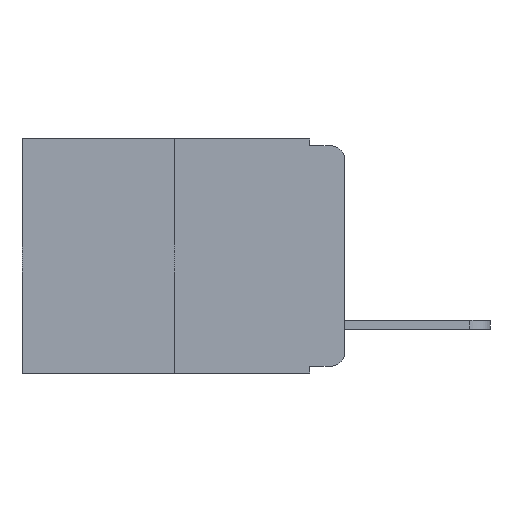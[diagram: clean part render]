
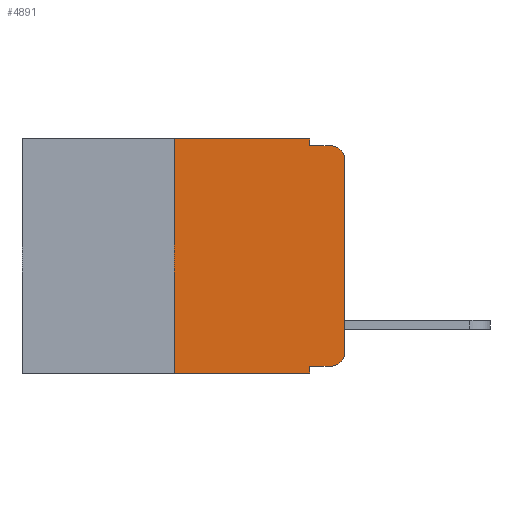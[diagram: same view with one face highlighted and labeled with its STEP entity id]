
A CAD part, left-side view. The second image highlights one B-rep face of the part: STEP entity #4891.
In plain terms, the highlighted planar face has unit normal (-1, 0, 0).
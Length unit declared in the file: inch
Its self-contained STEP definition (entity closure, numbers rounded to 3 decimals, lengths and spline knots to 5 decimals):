
#204 = LINE ( 'NONE', #1034, #8869 ) ;
#365 = EDGE_CURVE ( 'NONE', #8021, #4983, #11713, .T. ) ;
#414 = CARTESIAN_POINT ( 'NONE',  ( 0., 0., -0.313 ) ) ;
#567 = VECTOR ( 'NONE', #9850, 39.37008 ) ;
#837 = DIRECTION ( 'NONE',  ( -1., 0., 0. ) ) ;
#911 = VERTEX_POINT ( 'NONE', #12337 ) ;
#989 = VERTEX_POINT ( 'NONE', #10627 ) ;
#1034 = CARTESIAN_POINT ( 'NONE',  ( 0., 0.051, 0. ) ) ;
#1193 = ORIENTED_EDGE ( 'NONE', *, *, #3499, .T. ) ;
#1204 = EDGE_CURVE ( 'NONE', #8021, #5911, #12132, .T. ) ;
#1259 = PLANE ( 'NONE',  #11285 ) ;
#1434 = CARTESIAN_POINT ( 'NONE',  ( 0., 0.25, 0. ) ) ;
#1469 = ORIENTED_EDGE ( 'NONE', *, *, #8267, .T. ) ;
#1662 = DIRECTION ( 'NONE',  ( 0., -1., 0. ) ) ;
#1943 = CARTESIAN_POINT ( 'NONE',  ( 0., 0.473, 0. ) ) ;
#2091 = EDGE_CURVE ( 'NONE', #2557, #2866, #5139, .T. ) ;
#2169 = EDGE_CURVE ( 'NONE', #911, #7665, #3894, .T. ) ;
#2333 = DIRECTION ( 'NONE',  ( 1., 0., 0. ) ) ;
#2357 = EDGE_CURVE ( 'NONE', #7665, #2866, #12387, .T. ) ;
#2400 = DIRECTION ( 'NONE',  ( 0., 0., -1. ) ) ;
#2557 = VERTEX_POINT ( 'NONE', #4810 ) ;
#2712 = DIRECTION ( 'NONE',  ( 0., 0., -1. ) ) ;
#2798 = CARTESIAN_POINT ( 'NONE',  ( 0., 0., 0. ) ) ;
#2844 = VERTEX_POINT ( 'NONE', #4888 ) ;
#2866 = VERTEX_POINT ( 'NONE', #8182 ) ;
#3059 = CARTESIAN_POINT ( 'NONE',  ( 0., 0.25, 0. ) ) ;
#3358 = EDGE_CURVE ( 'NONE', #989, #2844, #4215, .T. ) ;
#3454 = EDGE_CURVE ( 'NONE', #989, #5911, #204, .T. ) ;
#3499 = EDGE_CURVE ( 'NONE', #2844, #7478, #7286, .T. ) ;
#3604 = CARTESIAN_POINT ( 'NONE',  ( 0., 0.051, -0.333 ) ) ;
#3894 = LINE ( 'NONE', #11073, #6180 ) ;
#4009 = CARTESIAN_POINT ( 'NONE',  ( 0., 0.473, -0.343 ) ) ;
#4024 = ORIENTED_EDGE ( 'NONE', *, *, #2357, .F. ) ;
#4215 = LINE ( 'NONE', #3604, #11380 ) ;
#4264 = VECTOR ( 'NONE', #5029, 39.37008 ) ;
#4461 = ORIENTED_EDGE ( 'NONE', *, *, #3358, .T. ) ;
#4555 = AXIS2_PLACEMENT_3D ( 'NONE', #12685, #11218, #11183 ) ;
#4810 = CARTESIAN_POINT ( 'NONE',  ( 0., 0., -0.03 ) ) ;
#4888 = CARTESIAN_POINT ( 'NONE',  ( 0., 0.02, -0.333 ) ) ;
#4891 = ADVANCED_FACE ( 'NONE', ( #7120 ), #1259, .F. ) ;
#4983 = VERTEX_POINT ( 'NONE', #1434 ) ;
#5029 = DIRECTION ( 'NONE',  ( 0., 0., 1. ) ) ;
#5051 = EDGE_LOOP ( 'NONE', ( #1469, #9804, #4024, #10085, #11496, #10766, #11885, #12178, #4461, #1193 ) ) ;
#5139 = CIRCLE ( 'NONE', #4555, 0.02 ) ;
#5370 = DIRECTION ( 'NONE',  ( 0., 0., -1. ) ) ;
#5911 = VERTEX_POINT ( 'NONE', #7107 ) ;
#5940 = LINE ( 'NONE', #2798, #567 ) ;
#6180 = VECTOR ( 'NONE', #5370, 39.37008 ) ;
#6460 = CARTESIAN_POINT ( 'NONE',  ( 0., 0.051, -0.01 ) ) ;
#6569 = AXIS2_PLACEMENT_3D ( 'NONE', #12702, #837, #2712 ) ;
#6968 = DIRECTION ( 'NONE',  ( 0., 0., -1. ) ) ;
#6973 = VECTOR ( 'NONE', #10863, 39.37008 ) ;
#6994 = VECTOR ( 'NONE', #10734, 39.37008 ) ;
#7107 = CARTESIAN_POINT ( 'NONE',  ( 0., 0.051, -0.343 ) ) ;
#7120 = FACE_OUTER_BOUND ( 'NONE', #5051, .T. ) ;
#7286 = CIRCLE ( 'NONE', #6569, 0.02 ) ;
#7478 = VERTEX_POINT ( 'NONE', #414 ) ;
#7665 = VERTEX_POINT ( 'NONE', #8048 ) ;
#8021 = VERTEX_POINT ( 'NONE', #10284 ) ;
#8048 = CARTESIAN_POINT ( 'NONE',  ( 0., 0.051, -0.01 ) ) ;
#8081 = DIRECTION ( 'NONE',  ( 0., -1., 0. ) ) ;
#8182 = CARTESIAN_POINT ( 'NONE',  ( 0., 0.02, -0.01 ) ) ;
#8267 = EDGE_CURVE ( 'NONE', #7478, #2557, #5940, .T. ) ;
#8869 = VECTOR ( 'NONE', #6968, 39.37008 ) ;
#9685 = VECTOR ( 'NONE', #8081, 39.37008 ) ;
#9804 = ORIENTED_EDGE ( 'NONE', *, *, #2091, .T. ) ;
#9850 = DIRECTION ( 'NONE',  ( 0., 0., 1. ) ) ;
#10085 = ORIENTED_EDGE ( 'NONE', *, *, #2169, .F. ) ;
#10284 = CARTESIAN_POINT ( 'NONE',  ( 0., 0.25, -0.343 ) ) ;
#10627 = CARTESIAN_POINT ( 'NONE',  ( 0., 0.051, -0.333 ) ) ;
#10734 = DIRECTION ( 'NONE',  ( 0., -1., 0. ) ) ;
#10766 = ORIENTED_EDGE ( 'NONE', *, *, #365, .F. ) ;
#10834 = CARTESIAN_POINT ( 'NONE',  ( 0., 0.473, 0. ) ) ;
#10863 = DIRECTION ( 'NONE',  ( 0., -1., 0. ) ) ;
#11073 = CARTESIAN_POINT ( 'NONE',  ( 0., 0.051, 0. ) ) ;
#11183 = DIRECTION ( 'NONE',  ( 0., 0., -1. ) ) ;
#11218 = DIRECTION ( 'NONE',  ( -1., 0., 0. ) ) ;
#11285 = AXIS2_PLACEMENT_3D ( 'NONE', #1943, #2333, #2400 ) ;
#11380 = VECTOR ( 'NONE', #1662, 39.37008 ) ;
#11496 = ORIENTED_EDGE ( 'NONE', *, *, #12577, .F. ) ;
#11713 = LINE ( 'NONE', #3059, #4264 ) ;
#11822 = LINE ( 'NONE', #10834, #6973 ) ;
#11885 = ORIENTED_EDGE ( 'NONE', *, *, #1204, .T. ) ;
#12132 = LINE ( 'NONE', #4009, #6994 ) ;
#12178 = ORIENTED_EDGE ( 'NONE', *, *, #3454, .F. ) ;
#12337 = CARTESIAN_POINT ( 'NONE',  ( 0., 0.051, 0. ) ) ;
#12387 = LINE ( 'NONE', #6460, #9685 ) ;
#12577 = EDGE_CURVE ( 'NONE', #4983, #911, #11822, .T. ) ;
#12685 = CARTESIAN_POINT ( 'NONE',  ( 0., 0.02, -0.03 ) ) ;
#12702 = CARTESIAN_POINT ( 'NONE',  ( 0., 0.02, -0.313 ) ) ;
